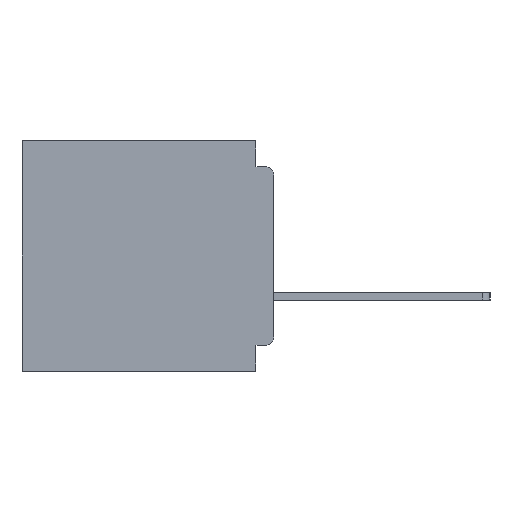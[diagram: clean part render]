
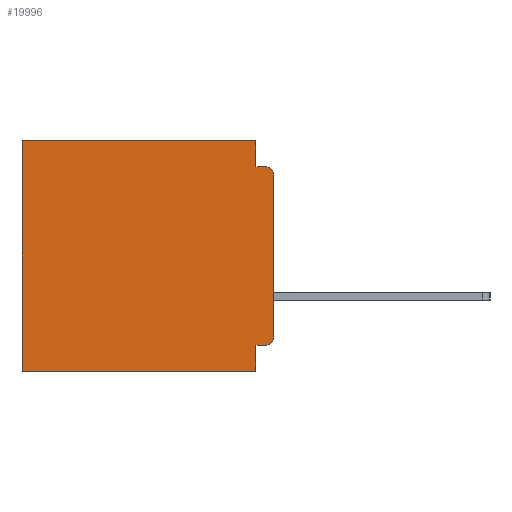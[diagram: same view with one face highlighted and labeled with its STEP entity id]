
A CAD part, left-side view. The second image highlights one B-rep face of the part: STEP entity #19996.
In plain terms, the highlighted planar face has unit normal (-1, 0, 0).
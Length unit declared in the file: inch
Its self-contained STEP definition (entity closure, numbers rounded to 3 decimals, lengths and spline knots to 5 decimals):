
#434 = ORIENTED_EDGE ( 'NONE', *, *, #18269, .F. ) ;
#864 = CARTESIAN_POINT ( 'NONE',  ( 0.3, 0.015, -0.355 ) ) ;
#1113 = PLANE ( 'NONE',  #38421 ) ;
#2012 = VECTOR ( 'NONE', #21148, 39.37008 ) ;
#2849 = ORIENTED_EDGE ( 'NONE', *, *, #18841, .F. ) ;
#3307 = ORIENTED_EDGE ( 'NONE', *, *, #20076, .F. ) ;
#3347 = ORIENTED_EDGE ( 'NONE', *, *, #13303, .F. ) ;
#4587 = CARTESIAN_POINT ( 'NONE',  ( 0.3, 0., -0.4 ) ) ;
#4647 = CARTESIAN_POINT ( 'NONE',  ( 0.3, 0.031, -0.4 ) ) ;
#5147 = LINE ( 'NONE', #4587, #28674 ) ;
#5718 = VERTEX_POINT ( 'NONE', #11350 ) ;
#5758 = CARTESIAN_POINT ( 'NONE',  ( 0.3, 0., 0. ) ) ;
#6207 = ORIENTED_EDGE ( 'NONE', *, *, #38099, .T. ) ;
#6241 = ORIENTED_EDGE ( 'NONE', *, *, #38329, .T. ) ;
#6727 = CARTESIAN_POINT ( 'NONE',  ( 0.3, 0., -0.34 ) ) ;
#6955 = CIRCLE ( 'NONE', #31070, 0.015 ) ;
#7936 = CARTESIAN_POINT ( 'NONE',  ( 0.3, 0.031, 0. ) ) ;
#7941 = VERTEX_POINT ( 'NONE', #11968 ) ;
#8327 = VERTEX_POINT ( 'NONE', #4647 ) ;
#8750 = CARTESIAN_POINT ( 'NONE',  ( 0.3, 0.031, -0.4 ) ) ;
#9189 = VECTOR ( 'NONE', #14274, 39.37008 ) ;
#9491 = VERTEX_POINT ( 'NONE', #6727 ) ;
#9570 = VECTOR ( 'NONE', #11021, 39.37008 ) ;
#9959 = EDGE_LOOP ( 'NONE', ( #3307, #6207, #34566, #2849, #27386, #29300, #434, #3347, #27865, #6241 ) ) ;
#10145 = LINE ( 'NONE', #20602, #9189 ) ;
#10458 = CARTESIAN_POINT ( 'NONE',  ( 0.3, 0.015, -0.045 ) ) ;
#11021 = DIRECTION ( 'NONE',  ( 0., 0., -1. ) ) ;
#11350 = CARTESIAN_POINT ( 'NONE',  ( 0.3, 0.437, 0. ) ) ;
#11467 = CARTESIAN_POINT ( 'NONE',  ( 0.3, 0.015, -0.34 ) ) ;
#11968 = CARTESIAN_POINT ( 'NONE',  ( 0.3, 0., -0.06 ) ) ;
#12395 = DIRECTION ( 'NONE',  ( 0., 0., -1. ) ) ;
#12710 = VECTOR ( 'NONE', #33434, 39.37008 ) ;
#13303 = EDGE_CURVE ( 'NONE', #17246, #8327, #26569, .T. ) ;
#13355 = DIRECTION ( 'NONE',  ( -1., 0., 0. ) ) ;
#13478 = DIRECTION ( 'NONE',  ( 1., 0., 0. ) ) ;
#13776 = VECTOR ( 'NONE', #12395, 39.37008 ) ;
#14274 = DIRECTION ( 'NONE',  ( 0., 1., 0. ) ) ;
#14567 = DIRECTION ( 'NONE',  ( 0., 0., -1. ) ) ;
#14751 = LINE ( 'NONE', #33862, #13776 ) ;
#15587 = EDGE_CURVE ( 'NONE', #32560, #31507, #28067, .T. ) ;
#16201 = EDGE_CURVE ( 'NONE', #37424, #5718, #30025, .T. ) ;
#16845 = CARTESIAN_POINT ( 'NONE',  ( 0.3, 0., -0.4 ) ) ;
#17246 = VERTEX_POINT ( 'NONE', #35240 ) ;
#17769 = LINE ( 'NONE', #7936, #9570 ) ;
#17847 = EDGE_CURVE ( 'NONE', #38077, #17246, #10145, .T. ) ;
#18269 = EDGE_CURVE ( 'NONE', #8327, #24369, #24578, .T. ) ;
#18841 = EDGE_CURVE ( 'NONE', #37424, #32560, #17769, .T. ) ;
#19996 = ADVANCED_FACE ( 'NONE', ( #23467 ), #1113, .F. ) ;
#20076 = EDGE_CURVE ( 'NONE', #7941, #9491, #5147, .T. ) ;
#20602 = CARTESIAN_POINT ( 'NONE',  ( 0.3, 0., -0.355 ) ) ;
#21148 = DIRECTION ( 'NONE',  ( 0., 0., -1. ) ) ;
#22849 = CIRCLE ( 'NONE', #24158, 0.015 ) ;
#23467 = FACE_OUTER_BOUND ( 'NONE', #9959, .T. ) ;
#23535 = CARTESIAN_POINT ( 'NONE',  ( 0.3, 0.031, 0. ) ) ;
#24140 = DIRECTION ( 'NONE',  ( 0., -1., 0. ) ) ;
#24158 = AXIS2_PLACEMENT_3D ( 'NONE', #11467, #32966, #14567 ) ;
#24274 = CARTESIAN_POINT ( 'NONE',  ( 0.3, 0., -0.045 ) ) ;
#24369 = VERTEX_POINT ( 'NONE', #38659 ) ;
#24578 = LINE ( 'NONE', #16845, #31742 ) ;
#24615 = CARTESIAN_POINT ( 'NONE',  ( 0.3, 0.031, -0.045 ) ) ;
#26569 = LINE ( 'NONE', #8750, #2012 ) ;
#26696 = EDGE_CURVE ( 'NONE', #5718, #24369, #14751, .T. ) ;
#27139 = VECTOR ( 'NONE', #24140, 39.37008 ) ;
#27386 = ORIENTED_EDGE ( 'NONE', *, *, #16201, .T. ) ;
#27865 = ORIENTED_EDGE ( 'NONE', *, *, #17847, .F. ) ;
#28067 = LINE ( 'NONE', #24274, #27139 ) ;
#28674 = VECTOR ( 'NONE', #35375, 39.37008 ) ;
#29053 = DIRECTION ( 'NONE',  ( 0., 1., 0. ) ) ;
#29300 = ORIENTED_EDGE ( 'NONE', *, *, #26696, .T. ) ;
#30025 = LINE ( 'NONE', #5758, #12710 ) ;
#31070 = AXIS2_PLACEMENT_3D ( 'NONE', #31761, #13355, #34846 ) ;
#31507 = VERTEX_POINT ( 'NONE', #10458 ) ;
#31742 = VECTOR ( 'NONE', #29053, 39.37008 ) ;
#31761 = CARTESIAN_POINT ( 'NONE',  ( 0.3, 0.015, -0.06 ) ) ;
#31888 = CARTESIAN_POINT ( 'NONE',  ( 0.3, 0., -0.4 ) ) ;
#32560 = VERTEX_POINT ( 'NONE', #24615 ) ;
#32966 = DIRECTION ( 'NONE',  ( -1., 0., 0. ) ) ;
#33434 = DIRECTION ( 'NONE',  ( 0., 1., 0. ) ) ;
#33862 = CARTESIAN_POINT ( 'NONE',  ( 0.3, 0.437, -0.4 ) ) ;
#34566 = ORIENTED_EDGE ( 'NONE', *, *, #15587, .F. ) ;
#34846 = DIRECTION ( 'NONE',  ( 0., 0., -1. ) ) ;
#34968 = DIRECTION ( 'NONE',  ( 0., 0., -1. ) ) ;
#35240 = CARTESIAN_POINT ( 'NONE',  ( 0.3, 0.031, -0.355 ) ) ;
#35375 = DIRECTION ( 'NONE',  ( 0., 0., -1. ) ) ;
#37424 = VERTEX_POINT ( 'NONE', #23535 ) ;
#38077 = VERTEX_POINT ( 'NONE', #864 ) ;
#38099 = EDGE_CURVE ( 'NONE', #7941, #31507, #6955, .T. ) ;
#38329 = EDGE_CURVE ( 'NONE', #38077, #9491, #22849, .T. ) ;
#38421 = AXIS2_PLACEMENT_3D ( 'NONE', #31888, #13478, #34968 ) ;
#38659 = CARTESIAN_POINT ( 'NONE',  ( 0.3, 0.437, -0.4 ) ) ;
